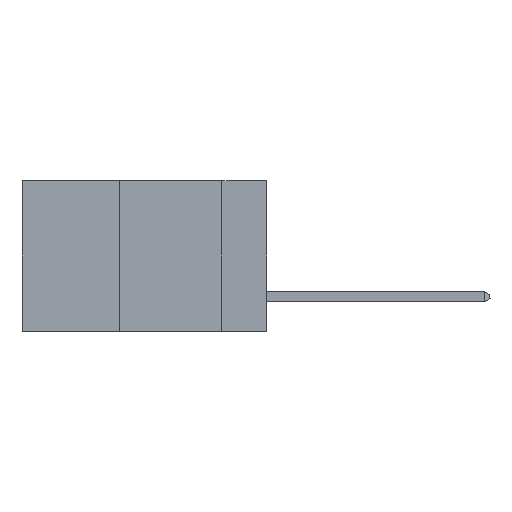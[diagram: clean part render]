
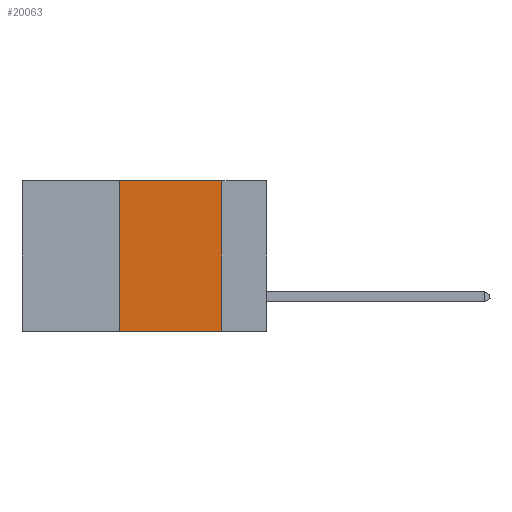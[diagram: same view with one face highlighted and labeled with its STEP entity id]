
A CAD part, left-side view. The second image highlights one B-rep face of the part: STEP entity #20063.
In plain terms, the highlighted planar face has unit normal (-1, 0, 0).
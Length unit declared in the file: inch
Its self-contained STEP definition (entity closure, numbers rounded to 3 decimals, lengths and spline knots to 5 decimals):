
#662 = ORIENTED_EDGE ( 'NONE', *, *, #9382, .F. ) ;
#782 = CARTESIAN_POINT ( 'NONE',  ( 0., 0.36, -0.37 ) ) ;
#1325 = VERTEX_POINT ( 'NONE', #9574 ) ;
#1454 = EDGE_CURVE ( 'NONE', #21590, #8499, #12971, .T. ) ;
#8499 = VERTEX_POINT ( 'NONE', #24280 ) ;
#8955 = AXIS2_PLACEMENT_3D ( 'NONE', #30963, #40459, #34649 ) ;
#9270 = DIRECTION ( 'NONE',  ( 0., -1., 0. ) ) ;
#9382 = EDGE_CURVE ( 'NONE', #1325, #8499, #32028, .T. ) ;
#9574 = CARTESIAN_POINT ( 'NONE',  ( 0., 0.11, 0. ) ) ;
#9648 = VECTOR ( 'NONE', #29376, 39.37008 ) ;
#10353 = DIRECTION ( 'NONE',  ( 0., -1., 0. ) ) ;
#12971 = LINE ( 'NONE', #16742, #33735 ) ;
#13551 = CARTESIAN_POINT ( 'NONE',  ( 0., 0.36, 0. ) ) ;
#14652 = LINE ( 'NONE', #22492, #9648 ) ;
#14816 = FACE_OUTER_BOUND ( 'NONE', #25803, .T. ) ;
#15115 = PLANE ( 'NONE',  #8955 ) ;
#16742 = CARTESIAN_POINT ( 'NONE',  ( 0., 0.6, -0.37 ) ) ;
#20063 = ADVANCED_FACE ( 'NONE', ( #14816 ), #15115, .F. ) ;
#20537 = DIRECTION ( 'NONE',  ( 0., 0., -1. ) ) ;
#21148 = EDGE_CURVE ( 'NONE', #32786, #1325, #40804, .T. ) ;
#21590 = VERTEX_POINT ( 'NONE', #782 ) ;
#22492 = CARTESIAN_POINT ( 'NONE',  ( 0., 0.36, 0. ) ) ;
#24280 = CARTESIAN_POINT ( 'NONE',  ( 0., 0.11, -0.37 ) ) ;
#25803 = EDGE_LOOP ( 'NONE', ( #662, #28400, #31038, #35428 ) ) ;
#28400 = ORIENTED_EDGE ( 'NONE', *, *, #21148, .F. ) ;
#29376 = DIRECTION ( 'NONE',  ( 0., 0., 1. ) ) ;
#30543 = VECTOR ( 'NONE', #20537, 39.37008 ) ;
#30573 = CARTESIAN_POINT ( 'NONE',  ( 0., 0.6, 0. ) ) ;
#30963 = CARTESIAN_POINT ( 'NONE',  ( 0., 0.6, 0. ) ) ;
#31038 = ORIENTED_EDGE ( 'NONE', *, *, #34939, .F. ) ;
#32028 = LINE ( 'NONE', #39417, #30543 ) ;
#32786 = VERTEX_POINT ( 'NONE', #13551 ) ;
#32908 = VECTOR ( 'NONE', #9270, 39.37008 ) ;
#33735 = VECTOR ( 'NONE', #10353, 39.37008 ) ;
#34649 = DIRECTION ( 'NONE',  ( 0., 0., -1. ) ) ;
#34939 = EDGE_CURVE ( 'NONE', #21590, #32786, #14652, .T. ) ;
#35428 = ORIENTED_EDGE ( 'NONE', *, *, #1454, .T. ) ;
#39417 = CARTESIAN_POINT ( 'NONE',  ( 0., 0.11, 0. ) ) ;
#40459 = DIRECTION ( 'NONE',  ( 1., 0., 0. ) ) ;
#40804 = LINE ( 'NONE', #30573, #32908 ) ;
